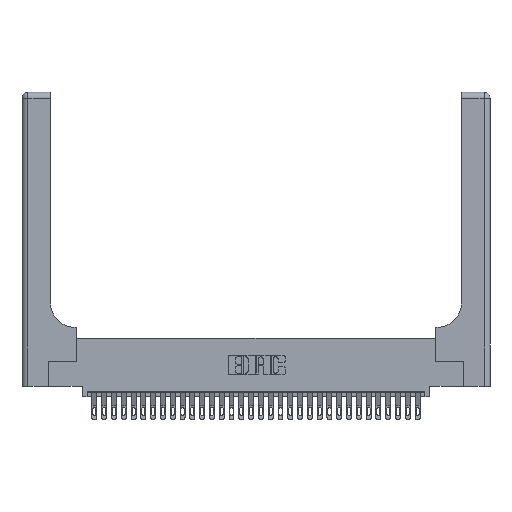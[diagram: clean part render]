
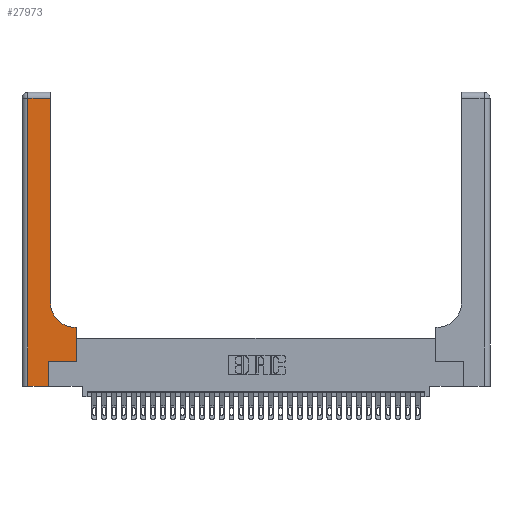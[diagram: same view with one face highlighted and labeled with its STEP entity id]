
A CAD part, top view. The second image highlights one B-rep face of the part: STEP entity #27973.
In plain terms, the highlighted planar face has unit normal (0, 0, 1).
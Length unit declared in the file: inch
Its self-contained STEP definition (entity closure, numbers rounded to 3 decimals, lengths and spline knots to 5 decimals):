
#161 = VERTEX_POINT ( 'NONE', #18525 ) ;
#513 = EDGE_CURVE ( 'NONE', #7663, #2439, #15444, .T. ) ;
#586 = CARTESIAN_POINT ( 'NONE',  ( 0.06, 3., 0.37 ) ) ;
#1490 = ORIENTED_EDGE ( 'NONE', *, *, #24631, .T. ) ;
#1536 = CIRCLE ( 'NONE', #12266, 0.25 ) ;
#1588 = CARTESIAN_POINT ( 'NONE',  ( 0.5415, 0.6, 0.37 ) ) ;
#1629 = LINE ( 'NONE', #32529, #21806 ) ;
#1696 = VECTOR ( 'NONE', #3735, 39.37008 ) ;
#2439 = VERTEX_POINT ( 'NONE', #5656 ) ;
#2734 = AXIS2_PLACEMENT_3D ( 'NONE', #3119, #8536, #16415 ) ;
#3119 = CARTESIAN_POINT ( 'NONE',  ( 0., 3., 0.37 ) ) ;
#3357 = CARTESIAN_POINT ( 'NONE',  ( 0.5585, 0.25, 0.37 ) ) ;
#3735 = DIRECTION ( 'NONE',  ( 1., 0., 0. ) ) ;
#3870 = VERTEX_POINT ( 'NONE', #6921 ) ;
#4285 = EDGE_LOOP ( 'NONE', ( #1490, #15876, #27165, #4534, #19784, #16623, #22725, #23139, #8266 ) ) ;
#4364 = VECTOR ( 'NONE', #28609, 39.37008 ) ;
#4534 = ORIENTED_EDGE ( 'NONE', *, *, #513, .T. ) ;
#5656 = CARTESIAN_POINT ( 'NONE',  ( 0.269, 0., 0.37 ) ) ;
#5796 = EDGE_CURVE ( 'NONE', #9651, #7663, #11257, .T. ) ;
#5993 = EDGE_CURVE ( 'NONE', #30081, #9331, #1536, .T. ) ;
#6260 = CARTESIAN_POINT ( 'NONE',  ( 0.5585, 0.6, 0.37 ) ) ;
#6921 = CARTESIAN_POINT ( 'NONE',  ( 0.269, 0.25, 0.37 ) ) ;
#7663 = VERTEX_POINT ( 'NONE', #31322 ) ;
#8266 = ORIENTED_EDGE ( 'NONE', *, *, #5993, .T. ) ;
#8536 = DIRECTION ( 'NONE',  ( 0., 0., -1. ) ) ;
#9331 = VERTEX_POINT ( 'NONE', #15342 ) ;
#9485 = CARTESIAN_POINT ( 'NONE',  ( 0.5415, 0.85, 0.37 ) ) ;
#9615 = LINE ( 'NONE', #3357, #4364 ) ;
#9651 = VERTEX_POINT ( 'NONE', #16322 ) ;
#10134 = EDGE_CURVE ( 'NONE', #3870, #161, #20534, .T. ) ;
#11257 = LINE ( 'NONE', #586, #16914 ) ;
#12044 = LINE ( 'NONE', #14387, #19266 ) ;
#12266 = AXIS2_PLACEMENT_3D ( 'NONE', #9485, #32480, #27530 ) ;
#12712 = CARTESIAN_POINT ( 'NONE',  ( 0.2915, 2.94, 0.37 ) ) ;
#13531 = VERTEX_POINT ( 'NONE', #12712 ) ;
#14003 = DIRECTION ( 'NONE',  ( 0., 1., 0. ) ) ;
#14169 = DIRECTION ( 'NONE',  ( -1., 0., 0. ) ) ;
#14387 = CARTESIAN_POINT ( 'NONE',  ( 0., 2.94, 0.37 ) ) ;
#14726 = LINE ( 'NONE', #22299, #19590 ) ;
#15212 = VERTEX_POINT ( 'NONE', #6260 ) ;
#15314 = VECTOR ( 'NONE', #14003, 39.37008 ) ;
#15342 = CARTESIAN_POINT ( 'NONE',  ( 0.2915, 0.85, 0.37 ) ) ;
#15444 = LINE ( 'NONE', #23910, #1696 ) ;
#15688 = LINE ( 'NONE', #24458, #15314 ) ;
#15876 = ORIENTED_EDGE ( 'NONE', *, *, #26251, .T. ) ;
#16322 = CARTESIAN_POINT ( 'NONE',  ( 0.06, 2.94, 0.37 ) ) ;
#16415 = DIRECTION ( 'NONE',  ( -1., 0., 0. ) ) ;
#16623 = ORIENTED_EDGE ( 'NONE', *, *, #10134, .T. ) ;
#16914 = VECTOR ( 'NONE', #21119, 39.37008 ) ;
#17564 = EDGE_CURVE ( 'NONE', #2439, #3870, #14726, .T. ) ;
#18525 = CARTESIAN_POINT ( 'NONE',  ( 0.5585, 0.25, 0.37 ) ) ;
#19266 = VECTOR ( 'NONE', #14169, 39.37008 ) ;
#19590 = VECTOR ( 'NONE', #19939, 39.37008 ) ;
#19784 = ORIENTED_EDGE ( 'NONE', *, *, #17564, .T. ) ;
#19939 = DIRECTION ( 'NONE',  ( 0., 1., 0. ) ) ;
#20534 = LINE ( 'NONE', #21043, #33045 ) ;
#20591 = EDGE_CURVE ( 'NONE', #15212, #30081, #1629, .T. ) ;
#21043 = CARTESIAN_POINT ( 'NONE',  ( 0.269, 0.25, 0.37 ) ) ;
#21119 = DIRECTION ( 'NONE',  ( 0., -1., 0. ) ) ;
#21806 = VECTOR ( 'NONE', #25094, 39.37008 ) ;
#21926 = EDGE_CURVE ( 'NONE', #161, #15212, #9615, .T. ) ;
#22299 = CARTESIAN_POINT ( 'NONE',  ( 0.269, 0., 0.37 ) ) ;
#22725 = ORIENTED_EDGE ( 'NONE', *, *, #21926, .T. ) ;
#23139 = ORIENTED_EDGE ( 'NONE', *, *, #20591, .T. ) ;
#23910 = CARTESIAN_POINT ( 'NONE',  ( 0., 0., 0.37 ) ) ;
#23954 = FACE_OUTER_BOUND ( 'NONE', #4285, .T. ) ;
#24458 = CARTESIAN_POINT ( 'NONE',  ( 0.2915, 3., 0.37 ) ) ;
#24631 = EDGE_CURVE ( 'NONE', #9331, #13531, #15688, .T. ) ;
#25094 = DIRECTION ( 'NONE',  ( -1., 0., 0. ) ) ;
#26251 = EDGE_CURVE ( 'NONE', #13531, #9651, #12044, .T. ) ;
#26689 = PLANE ( 'NONE',  #2734 ) ;
#27165 = ORIENTED_EDGE ( 'NONE', *, *, #5796, .T. ) ;
#27530 = DIRECTION ( 'NONE',  ( 1., 0., 0. ) ) ;
#27973 = ADVANCED_FACE ( 'NONE', ( #23954 ), #26689, .F. ) ;
#28609 = DIRECTION ( 'NONE',  ( 0., 1., 0. ) ) ;
#30081 = VERTEX_POINT ( 'NONE', #1588 ) ;
#31322 = CARTESIAN_POINT ( 'NONE',  ( 0.06, 0., 0.37 ) ) ;
#31516 = DIRECTION ( 'NONE',  ( 1., 0., 0. ) ) ;
#32480 = DIRECTION ( 'NONE',  ( 0., 0., -1. ) ) ;
#32529 = CARTESIAN_POINT ( 'NONE',  ( 0.2915, 0.6, 0.37 ) ) ;
#33045 = VECTOR ( 'NONE', #31516, 39.37008 ) ;
